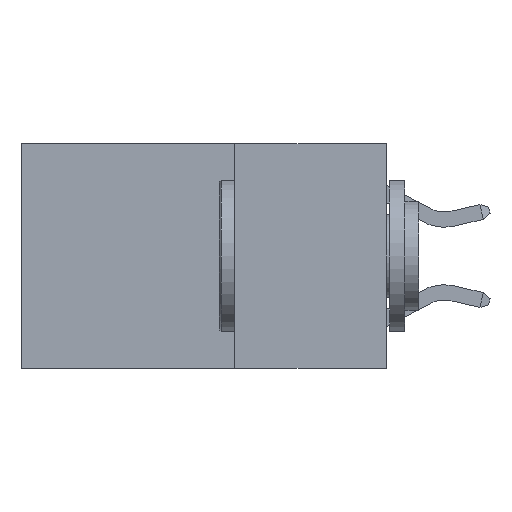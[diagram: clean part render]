
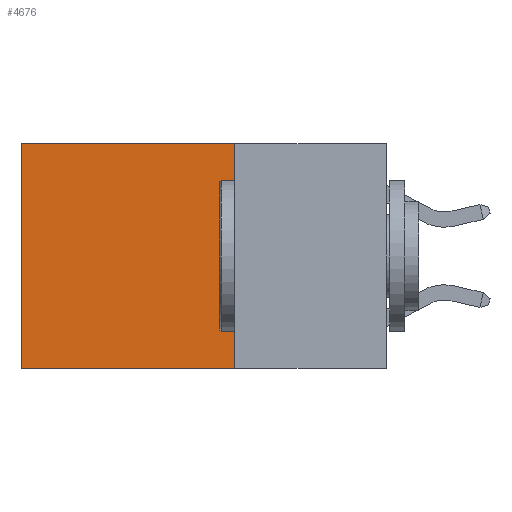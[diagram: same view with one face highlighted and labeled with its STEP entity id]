
A CAD part, left-side view. The second image highlights one B-rep face of the part: STEP entity #4676.
In plain terms, the highlighted planar face has unit normal (-1, 0, 0).
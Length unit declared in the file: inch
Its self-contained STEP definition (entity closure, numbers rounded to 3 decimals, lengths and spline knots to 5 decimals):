
#598 = CARTESIAN_POINT ( 'NONE',  ( 0.2625, 0.6, 0. ) ) ;
#679 = CARTESIAN_POINT ( 'NONE',  ( 0.2625, 0.25, 0. ) ) ;
#941 = ORIENTED_EDGE ( 'NONE', *, *, #5930, .F. ) ;
#964 = LINE ( 'NONE', #679, #8326 ) ;
#1535 = ORIENTED_EDGE ( 'NONE', *, *, #19246, .F. ) ;
#2254 = CARTESIAN_POINT ( 'NONE',  ( 0.2625, 0.25, 0. ) ) ;
#3510 = VERTEX_POINT ( 'NONE', #4276 ) ;
#4276 = CARTESIAN_POINT ( 'NONE',  ( 0.2625, 0.6, 0. ) ) ;
#4676 = ADVANCED_FACE ( 'NONE', ( #5265 ), #5069, .F. ) ;
#4735 = CARTESIAN_POINT ( 'NONE',  ( 0.2625, 0.25, -0.37 ) ) ;
#5069 = PLANE ( 'NONE',  #8395 ) ;
#5265 = FACE_OUTER_BOUND ( 'NONE', #9071, .T. ) ;
#5351 = VECTOR ( 'NONE', #15035, 39.37008 ) ;
#5894 = ORIENTED_EDGE ( 'NONE', *, *, #6725, .T. ) ;
#5930 = EDGE_CURVE ( 'NONE', #6355, #8576, #16525, .T. ) ;
#6355 = VERTEX_POINT ( 'NONE', #6949 ) ;
#6650 = EDGE_CURVE ( 'NONE', #3510, #8576, #10997, .T. ) ;
#6725 = EDGE_CURVE ( 'NONE', #19297, #3510, #14789, .T. ) ;
#6949 = CARTESIAN_POINT ( 'NONE',  ( 0.2625, 0.25, -0.37 ) ) ;
#7020 = DIRECTION ( 'NONE',  ( 0., 0., -1. ) ) ;
#8326 = VECTOR ( 'NONE', #7020, 39.37008 ) ;
#8395 = AXIS2_PLACEMENT_3D ( 'NONE', #9876, #17243, #14183 ) ;
#8427 = CARTESIAN_POINT ( 'NONE',  ( 0.2625, 0.25, 0. ) ) ;
#8576 = VERTEX_POINT ( 'NONE', #19118 ) ;
#9071 = EDGE_LOOP ( 'NONE', ( #17090, #941, #1535, #5894 ) ) ;
#9876 = CARTESIAN_POINT ( 'NONE',  ( 0.2625, 0.25, 0. ) ) ;
#10713 = VECTOR ( 'NONE', #14504, 39.37008 ) ;
#10997 = LINE ( 'NONE', #598, #11036 ) ;
#11036 = VECTOR ( 'NONE', #18566, 39.37008 ) ;
#14183 = DIRECTION ( 'NONE',  ( 0., 0., -1. ) ) ;
#14504 = DIRECTION ( 'NONE',  ( 0., 1., 0. ) ) ;
#14789 = LINE ( 'NONE', #8427, #10713 ) ;
#15035 = DIRECTION ( 'NONE',  ( 0., 1., 0. ) ) ;
#16525 = LINE ( 'NONE', #4735, #5351 ) ;
#17090 = ORIENTED_EDGE ( 'NONE', *, *, #6650, .T. ) ;
#17243 = DIRECTION ( 'NONE',  ( 1., 0., 0. ) ) ;
#18566 = DIRECTION ( 'NONE',  ( 0., 0., -1. ) ) ;
#19118 = CARTESIAN_POINT ( 'NONE',  ( 0.2625, 0.6, -0.37 ) ) ;
#19246 = EDGE_CURVE ( 'NONE', #19297, #6355, #964, .T. ) ;
#19297 = VERTEX_POINT ( 'NONE', #2254 ) ;
